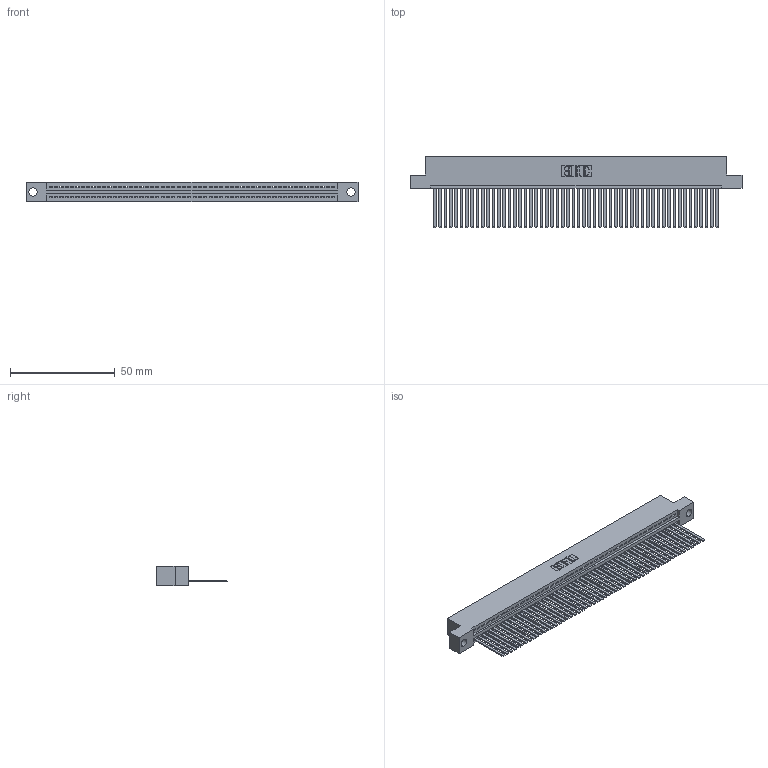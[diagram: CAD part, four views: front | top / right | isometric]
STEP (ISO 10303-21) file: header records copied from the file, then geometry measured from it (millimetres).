
FILE_DESCRIPTION (( 'STEP AP203' ), '1' );
FILE_NAME ('345-054-544-104.STEP', '2019-10-10T00:42:04', ( '' ), ( '' ), 'SwSTEP 2.0', 'SolidWorks 2016', '' );
FILE_SCHEMA (( 'CONFIG_CONTROL_DESIGN' ));
Length unit declared in the file: inch
Products named in the file (3): 345 Part_Flush Mounting Lugs - 0.156 Dia-TH; 345-292-001_345-293-144; 345-054-544-104
Assembly tree (55 placements, depth 2):
  345-054-544-104
    345 Part_Flush Mounting Lugs - 0.156 Dia-TH
    345-292-001_345-293-144  x54
Bounding box: 158.37 x 33.96 x 9.4 mm (x, y, z)
Volume: 15677.9 mm3; surface area: 22683.8 mm2
Topology: 55 solids, 55 shells, 2934 faces, 8873 edges, 5842 vertices
Faces by surface type: plane 2024, cylinder 910
Entity records: 38845 total; most frequent: CARTESIAN_POINT 6734, ORIENTED_EDGE 6722, DIRECTION 5861, EDGE_CURVE 3361, VECTOR 3017, LINE 3017, VERTEX_POINT 2238, AXIS2_PLACEMENT_3D 1422
